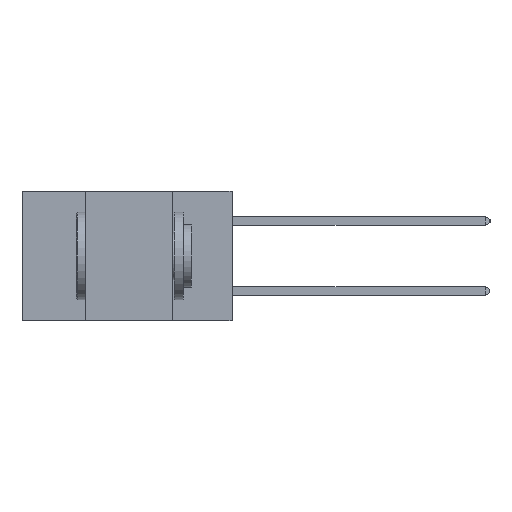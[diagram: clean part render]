
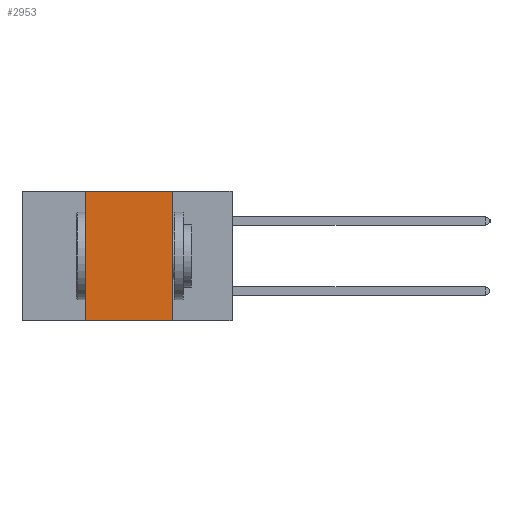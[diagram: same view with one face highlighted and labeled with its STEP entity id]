
A CAD part, left-side view. The second image highlights one B-rep face of the part: STEP entity #2953.
In plain terms, the highlighted planar face has unit normal (-1, 0, 0).
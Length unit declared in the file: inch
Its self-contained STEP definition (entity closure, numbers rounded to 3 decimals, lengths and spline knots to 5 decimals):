
#272 = DIRECTION ( 'NONE',  ( 0., -1., 0. ) ) ;
#854 = AXIS2_PLACEMENT_3D ( 'NONE', #13055, #12805, #12792 ) ;
#1058 = EDGE_CURVE ( 'NONE', #13794, #5961, #10935, .T. ) ;
#2010 = CARTESIAN_POINT ( 'NONE',  ( 0., 0.17, -0.37 ) ) ;
#2431 = CARTESIAN_POINT ( 'NONE',  ( 0., 0.6, 0. ) ) ;
#2953 = ADVANCED_FACE ( 'NONE', ( #6497 ), #12895, .F. ) ;
#4162 = CARTESIAN_POINT ( 'NONE',  ( 0., 0.42, 0. ) ) ;
#4339 = CARTESIAN_POINT ( 'NONE',  ( 0., 0.42, -0.37 ) ) ;
#4777 = EDGE_CURVE ( 'NONE', #4779, #13794, #6276, .T. ) ;
#4779 = VERTEX_POINT ( 'NONE', #8029 ) ;
#5047 = VECTOR ( 'NONE', #272, 39.37008 ) ;
#5809 = CARTESIAN_POINT ( 'NONE',  ( 0., 0.6, -0.37 ) ) ;
#5961 = VERTEX_POINT ( 'NONE', #2010 ) ;
#6010 = VERTEX_POINT ( 'NONE', #4339 ) ;
#6276 = LINE ( 'NONE', #2431, #8849 ) ;
#6497 = FACE_OUTER_BOUND ( 'NONE', #9892, .T. ) ;
#6613 = DIRECTION ( 'NONE',  ( 0., 0., 1. ) ) ;
#7318 = ORIENTED_EDGE ( 'NONE', *, *, #4777, .F. ) ;
#7781 = VECTOR ( 'NONE', #6613, 39.37008 ) ;
#7876 = CARTESIAN_POINT ( 'NONE',  ( 0., 0.17, 0. ) ) ;
#7950 = LINE ( 'NONE', #5809, #5047 ) ;
#8029 = CARTESIAN_POINT ( 'NONE',  ( 0., 0.42, 0. ) ) ;
#8139 = LINE ( 'NONE', #4162, #7781 ) ;
#8370 = ORIENTED_EDGE ( 'NONE', *, *, #13666, .F. ) ;
#8849 = VECTOR ( 'NONE', #11255, 39.37008 ) ;
#9835 = ORIENTED_EDGE ( 'NONE', *, *, #1058, .F. ) ;
#9892 = EDGE_LOOP ( 'NONE', ( #9835, #7318, #8370, #10037 ) ) ;
#10037 = ORIENTED_EDGE ( 'NONE', *, *, #13888, .T. ) ;
#10935 = LINE ( 'NONE', #13534, #13412 ) ;
#11255 = DIRECTION ( 'NONE',  ( 0., -1., 0. ) ) ;
#12792 = DIRECTION ( 'NONE',  ( 0., 0., -1. ) ) ;
#12805 = DIRECTION ( 'NONE',  ( 1., 0., 0. ) ) ;
#12895 = PLANE ( 'NONE',  #854 ) ;
#13055 = CARTESIAN_POINT ( 'NONE',  ( 0., 0.6, 0. ) ) ;
#13412 = VECTOR ( 'NONE', #13589, 39.37008 ) ;
#13534 = CARTESIAN_POINT ( 'NONE',  ( 0., 0.17, 0. ) ) ;
#13589 = DIRECTION ( 'NONE',  ( 0., 0., -1. ) ) ;
#13666 = EDGE_CURVE ( 'NONE', #6010, #4779, #8139, .T. ) ;
#13794 = VERTEX_POINT ( 'NONE', #7876 ) ;
#13888 = EDGE_CURVE ( 'NONE', #6010, #5961, #7950, .T. ) ;
